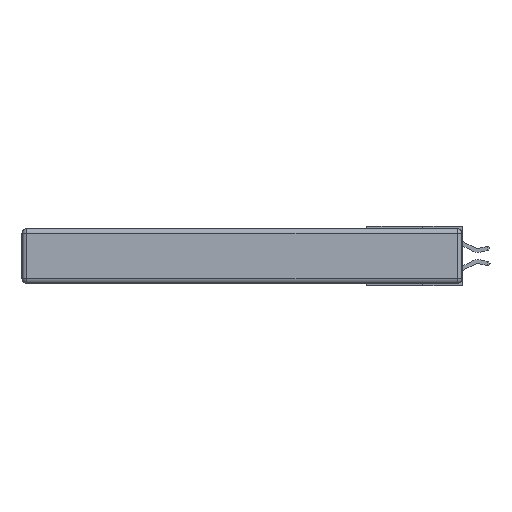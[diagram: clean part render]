
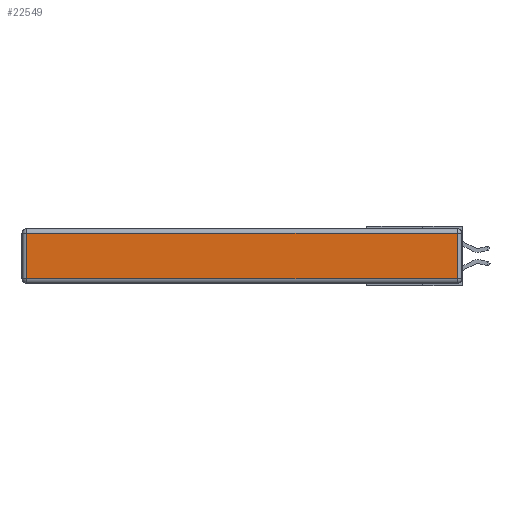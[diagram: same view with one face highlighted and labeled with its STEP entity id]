
A CAD part, left-side view. The second image highlights one B-rep face of the part: STEP entity #22549.
In plain terms, the highlighted planar face has unit normal (-1, 0, 0).
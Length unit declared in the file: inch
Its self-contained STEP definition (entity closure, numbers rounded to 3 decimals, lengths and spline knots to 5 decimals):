
#341 = FACE_OUTER_BOUND ( 'NONE', #16027, .T. ) ;
#738 = CARTESIAN_POINT ( 'NONE',  ( 0., 2.72, -0.343 ) ) ;
#908 = ORIENTED_EDGE ( 'NONE', *, *, #14606, .T. ) ;
#991 = VERTEX_POINT ( 'NONE', #4181 ) ;
#2272 = ORIENTED_EDGE ( 'NONE', *, *, #19214, .T. ) ;
#2424 = DIRECTION ( 'NONE',  ( 0., 1., 0. ) ) ;
#4181 = CARTESIAN_POINT ( 'NONE',  ( 0., 2.72, -0.03 ) ) ;
#5424 = PLANE ( 'NONE',  #15574 ) ;
#6196 = DIRECTION ( 'NONE',  ( 0., 0., -1. ) ) ;
#6895 = CARTESIAN_POINT ( 'NONE',  ( 0., 0.03, -0.313 ) ) ;
#7537 = EDGE_CURVE ( 'NONE', #9429, #30687, #16782, .T. ) ;
#7886 = ORIENTED_EDGE ( 'NONE', *, *, #27380, .T. ) ;
#9339 = VERTEX_POINT ( 'NONE', #25968 ) ;
#9429 = VERTEX_POINT ( 'NONE', #6895 ) ;
#11023 = LINE ( 'NONE', #13373, #30889 ) ;
#11471 = VECTOR ( 'NONE', #6196, 39.37008 ) ;
#13373 = CARTESIAN_POINT ( 'NONE',  ( 0., 0., -0.313 ) ) ;
#14606 = EDGE_CURVE ( 'NONE', #9339, #9429, #11023, .T. ) ;
#14715 = ORIENTED_EDGE ( 'NONE', *, *, #7537, .T. ) ;
#14996 = LINE ( 'NONE', #25853, #17824 ) ;
#15574 = AXIS2_PLACEMENT_3D ( 'NONE', #16078, #20928, #31639 ) ;
#16027 = EDGE_LOOP ( 'NONE', ( #908, #14715, #7886, #2272 ) ) ;
#16078 = CARTESIAN_POINT ( 'NONE',  ( 0., 0., -0.343 ) ) ;
#16110 = CARTESIAN_POINT ( 'NONE',  ( 0., 0.03, -0.03 ) ) ;
#16782 = LINE ( 'NONE', #29087, #21242 ) ;
#17824 = VECTOR ( 'NONE', #2424, 39.37008 ) ;
#19214 = EDGE_CURVE ( 'NONE', #991, #9339, #32191, .T. ) ;
#20928 = DIRECTION ( 'NONE',  ( -1., 0., 0. ) ) ;
#21242 = VECTOR ( 'NONE', #24116, 39.37008 ) ;
#22549 = ADVANCED_FACE ( 'NONE', ( #341 ), #5424, .T. ) ;
#23716 = DIRECTION ( 'NONE',  ( 0., -1., 0. ) ) ;
#24116 = DIRECTION ( 'NONE',  ( 0., 0., 1. ) ) ;
#25853 = CARTESIAN_POINT ( 'NONE',  ( 0., 2.75, -0.03 ) ) ;
#25968 = CARTESIAN_POINT ( 'NONE',  ( 0., 2.72, -0.313 ) ) ;
#27380 = EDGE_CURVE ( 'NONE', #30687, #991, #14996, .T. ) ;
#29087 = CARTESIAN_POINT ( 'NONE',  ( 0., 0.03, -0.343 ) ) ;
#30687 = VERTEX_POINT ( 'NONE', #16110 ) ;
#30889 = VECTOR ( 'NONE', #23716, 39.37008 ) ;
#31639 = DIRECTION ( 'NONE',  ( 0., 0., 1. ) ) ;
#32191 = LINE ( 'NONE', #738, #11471 ) ;
